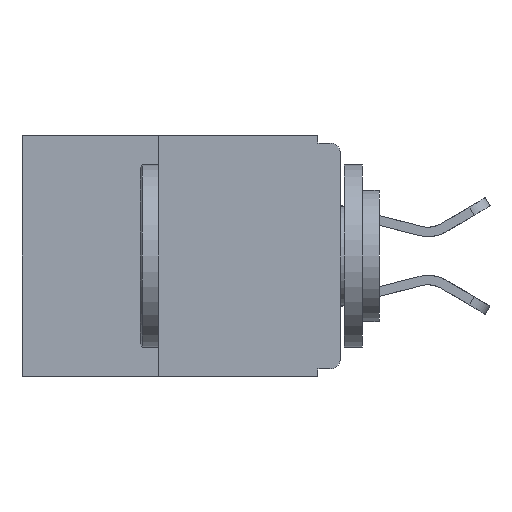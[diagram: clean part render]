
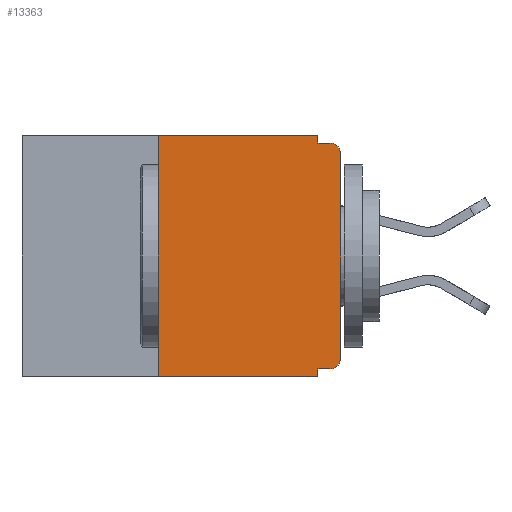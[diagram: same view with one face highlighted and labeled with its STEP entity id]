
A CAD part, left-side view. The second image highlights one B-rep face of the part: STEP entity #13363.
In plain terms, the highlighted planar face has unit normal (-1, 0, 0).
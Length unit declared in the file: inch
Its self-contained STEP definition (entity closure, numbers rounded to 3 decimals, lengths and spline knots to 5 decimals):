
#138 = CARTESIAN_POINT ( 'NONE',  ( 0., 0.031, 0. ) ) ;
#467 = DIRECTION ( 'NONE',  ( -1., 0., 0. ) ) ;
#741 = CIRCLE ( 'NONE', #24870, 0.015 ) ;
#1211 = CARTESIAN_POINT ( 'NONE',  ( 0., 0., -0.305 ) ) ;
#1898 = VERTEX_POINT ( 'NONE', #11022 ) ;
#2011 = EDGE_CURVE ( 'NONE', #20161, #1898, #3436, .T. ) ;
#2099 = DIRECTION ( 'NONE',  ( 0., 0., -1. ) ) ;
#2653 = CARTESIAN_POINT ( 'NONE',  ( 0., 0.031, -0.32 ) ) ;
#2761 = EDGE_LOOP ( 'NONE', ( #24248, #24796, #24974, #26825, #30614, #5255, #10279, #12432, #12667, #13310 ) ) ;
#3302 = LINE ( 'NONE', #138, #16055 ) ;
#3339 = CARTESIAN_POINT ( 'NONE',  ( 0., 0., -0.32 ) ) ;
#3436 = LINE ( 'NONE', #4715, #9095 ) ;
#4616 = EDGE_CURVE ( 'NONE', #18758, #26752, #19966, .T. ) ;
#4715 = CARTESIAN_POINT ( 'NONE',  ( 0., 0.25, -0.33 ) ) ;
#5056 = DIRECTION ( 'NONE',  ( 0., -1., 0. ) ) ;
#5255 = ORIENTED_EDGE ( 'NONE', *, *, #2011, .F. ) ;
#7096 = VERTEX_POINT ( 'NONE', #18641 ) ;
#7984 = VERTEX_POINT ( 'NONE', #22518 ) ;
#9078 = DIRECTION ( 'NONE',  ( 0., 0., -1. ) ) ;
#9095 = VECTOR ( 'NONE', #23984, 39.37008 ) ;
#9120 = DIRECTION ( 'NONE',  ( -1., 0., 0. ) ) ;
#9150 = CARTESIAN_POINT ( 'NONE',  ( 0., 0.015, -0.025 ) ) ;
#9259 = DIRECTION ( 'NONE',  ( 0., 0., 1. ) ) ;
#10279 = ORIENTED_EDGE ( 'NONE', *, *, #24084, .T. ) ;
#10394 = VECTOR ( 'NONE', #2099, 39.37008 ) ;
#10860 = CARTESIAN_POINT ( 'NONE',  ( 0., 0.25, -0.33 ) ) ;
#11022 = CARTESIAN_POINT ( 'NONE',  ( 0., 0.25, 0. ) ) ;
#11326 = EDGE_CURVE ( 'NONE', #13245, #12765, #741, .T. ) ;
#11511 = CARTESIAN_POINT ( 'NONE',  ( 0., 0.437, 0. ) ) ;
#12432 = ORIENTED_EDGE ( 'NONE', *, *, #15192, .F. ) ;
#12667 = ORIENTED_EDGE ( 'NONE', *, *, #16168, .F. ) ;
#12765 = VERTEX_POINT ( 'NONE', #1211 ) ;
#12961 = EDGE_CURVE ( 'NONE', #12765, #18758, #14653, .T. ) ;
#13078 = CARTESIAN_POINT ( 'NONE',  ( 0., 0.015, -0.01 ) ) ;
#13245 = VERTEX_POINT ( 'NONE', #26733 ) ;
#13310 = ORIENTED_EDGE ( 'NONE', *, *, #11326, .T. ) ;
#13363 = ADVANCED_FACE ( 'NONE', ( #30057 ), #27161, .F. ) ;
#13924 = VECTOR ( 'NONE', #5056, 39.37008 ) ;
#14285 = EDGE_CURVE ( 'NONE', #7096, #24665, #3302, .T. ) ;
#14653 = LINE ( 'NONE', #23514, #21764 ) ;
#14671 = LINE ( 'NONE', #28672, #13924 ) ;
#14925 = CARTESIAN_POINT ( 'NONE',  ( 0., 0.015, -0.305 ) ) ;
#14949 = CARTESIAN_POINT ( 'NONE',  ( 0., 0.031, -0.01 ) ) ;
#15192 = EDGE_CURVE ( 'NONE', #18017, #7984, #23052, .T. ) ;
#15403 = DIRECTION ( 'NONE',  ( 0., 0., -1. ) ) ;
#16055 = VECTOR ( 'NONE', #17000, 39.37008 ) ;
#16168 = EDGE_CURVE ( 'NONE', #13245, #18017, #29661, .T. ) ;
#16456 = CARTESIAN_POINT ( 'NONE',  ( 0., 0., -0.01 ) ) ;
#17000 = DIRECTION ( 'NONE',  ( 0., 0., -1. ) ) ;
#17321 = DIRECTION ( 'NONE',  ( 0., 0., -1. ) ) ;
#18017 = VERTEX_POINT ( 'NONE', #2653 ) ;
#18641 = CARTESIAN_POINT ( 'NONE',  ( 0., 0.031, 0. ) ) ;
#18707 = DIRECTION ( 'NONE',  ( 0., -1., 0. ) ) ;
#18758 = VERTEX_POINT ( 'NONE', #24419 ) ;
#18904 = CARTESIAN_POINT ( 'NONE',  ( 0., 0.031, -0.33 ) ) ;
#19905 = VECTOR ( 'NONE', #30490, 39.37008 ) ;
#19966 = CIRCLE ( 'NONE', #25728, 0.015 ) ;
#20107 = DIRECTION ( 'NONE',  ( 0., 1., 0. ) ) ;
#20161 = VERTEX_POINT ( 'NONE', #10860 ) ;
#21764 = VECTOR ( 'NONE', #9259, 39.37008 ) ;
#22398 = AXIS2_PLACEMENT_3D ( 'NONE', #22472, #29470, #15403 ) ;
#22472 = CARTESIAN_POINT ( 'NONE',  ( 0., 0.437, 0. ) ) ;
#22518 = CARTESIAN_POINT ( 'NONE',  ( 0., 0.031, -0.33 ) ) ;
#23009 = VECTOR ( 'NONE', #18707, 39.37008 ) ;
#23052 = LINE ( 'NONE', #18904, #10394 ) ;
#23514 = CARTESIAN_POINT ( 'NONE',  ( 0., 0., 0. ) ) ;
#23984 = DIRECTION ( 'NONE',  ( 0., 0., 1. ) ) ;
#24084 = EDGE_CURVE ( 'NONE', #20161, #7984, #14671, .T. ) ;
#24248 = ORIENTED_EDGE ( 'NONE', *, *, #12961, .T. ) ;
#24419 = CARTESIAN_POINT ( 'NONE',  ( 0., 0., -0.025 ) ) ;
#24665 = VERTEX_POINT ( 'NONE', #14949 ) ;
#24796 = ORIENTED_EDGE ( 'NONE', *, *, #4616, .T. ) ;
#24870 = AXIS2_PLACEMENT_3D ( 'NONE', #14925, #467, #17321 ) ;
#24974 = ORIENTED_EDGE ( 'NONE', *, *, #29276, .F. ) ;
#25728 = AXIS2_PLACEMENT_3D ( 'NONE', #9150, #9120, #9078 ) ;
#26091 = LINE ( 'NONE', #16456, #19905 ) ;
#26733 = CARTESIAN_POINT ( 'NONE',  ( 0., 0.015, -0.32 ) ) ;
#26752 = VERTEX_POINT ( 'NONE', #13078 ) ;
#26825 = ORIENTED_EDGE ( 'NONE', *, *, #14285, .F. ) ;
#26979 = EDGE_CURVE ( 'NONE', #1898, #7096, #28483, .T. ) ;
#27161 = PLANE ( 'NONE',  #22398 ) ;
#28483 = LINE ( 'NONE', #11511, #23009 ) ;
#28672 = CARTESIAN_POINT ( 'NONE',  ( 0., 0.437, -0.33 ) ) ;
#28930 = VECTOR ( 'NONE', #20107, 39.37008 ) ;
#29276 = EDGE_CURVE ( 'NONE', #24665, #26752, #26091, .T. ) ;
#29470 = DIRECTION ( 'NONE',  ( 1., 0., 0. ) ) ;
#29661 = LINE ( 'NONE', #3339, #28930 ) ;
#30057 = FACE_OUTER_BOUND ( 'NONE', #2761, .T. ) ;
#30490 = DIRECTION ( 'NONE',  ( 0., -1., 0. ) ) ;
#30614 = ORIENTED_EDGE ( 'NONE', *, *, #26979, .F. ) ;
